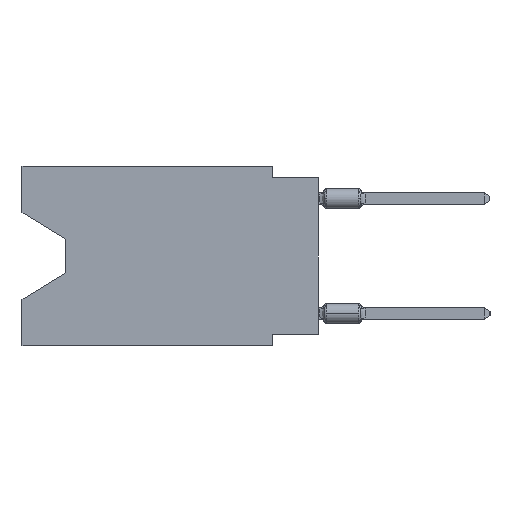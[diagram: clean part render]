
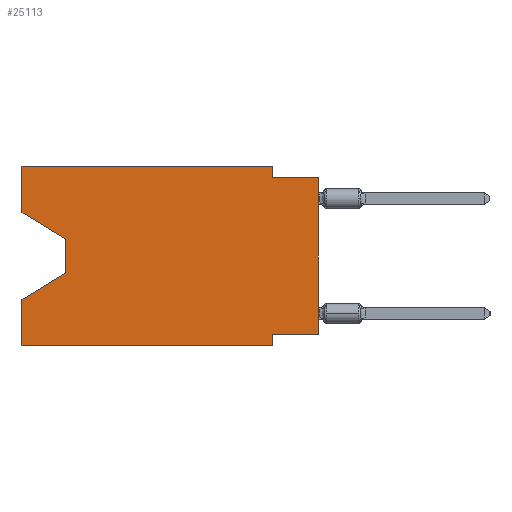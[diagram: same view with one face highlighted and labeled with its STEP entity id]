
A CAD part, left-side view. The second image highlights one B-rep face of the part: STEP entity #25113.
In plain terms, the highlighted planar face has unit normal (-1, 0, 0).
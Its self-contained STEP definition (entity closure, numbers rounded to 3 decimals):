
#298 = LINE ( 'NONE', #15007, #31494 ) ;
#526 = VERTEX_POINT ( 'NONE', #36395 ) ;
#696 = VECTOR ( 'NONE', #44986, 1000. ) ;
#1063 = VECTOR ( 'NONE', #20297, 1000. ) ;
#1226 = DIRECTION ( 'NONE',  ( 0., -1., 0. ) ) ;
#1375 = DIRECTION ( 'NONE',  ( 0., 0., -1. ) ) ;
#2373 = CARTESIAN_POINT ( 'NONE',  ( 0., 16.383, -9.906 ) ) ;
#3007 = LINE ( 'NONE', #8587, #31546 ) ;
#3595 = EDGE_CURVE ( 'NONE', #54115, #43270, #24095, .T. ) ;
#3749 = CARTESIAN_POINT ( 'NONE',  ( 0., 13.97, -4.013 ) ) ;
#4097 = CARTESIAN_POINT ( 'NONE',  ( 0., 16.383, 0. ) ) ;
#4429 = VERTEX_POINT ( 'NONE', #20169 ) ;
#4543 = VERTEX_POINT ( 'NONE', #36067 ) ;
#6307 = EDGE_CURVE ( 'NONE', #28124, #10658, #19996, .T. ) ;
#7804 = EDGE_CURVE ( 'NONE', #526, #4543, #36896, .T. ) ;
#8149 = CARTESIAN_POINT ( 'NONE',  ( 0., 16.383, -7.36 ) ) ;
#8587 = CARTESIAN_POINT ( 'NONE',  ( 0., 13.97, -5.893 ) ) ;
#8866 = VERTEX_POINT ( 'NONE', #20973 ) ;
#9098 = VERTEX_POINT ( 'NONE', #19689 ) ;
#9407 = EDGE_CURVE ( 'NONE', #526, #4429, #37939, .T. ) ;
#10426 = PLANE ( 'NONE',  #21625 ) ;
#10658 = VERTEX_POINT ( 'NONE', #36509 ) ;
#11030 = DIRECTION ( 'NONE',  ( 0., 0., -1. ) ) ;
#11902 = EDGE_CURVE ( 'NONE', #4543, #22830, #56758, .T. ) ;
#13470 = ORIENTED_EDGE ( 'NONE', *, *, #57463, .T. ) ;
#13638 = ORIENTED_EDGE ( 'NONE', *, *, #9407, .T. ) ;
#14748 = VERTEX_POINT ( 'NONE', #20993 ) ;
#15007 = CARTESIAN_POINT ( 'NONE',  ( 0., 2.54, 0. ) ) ;
#16032 = VECTOR ( 'NONE', #37025, 1000. ) ;
#18238 = CARTESIAN_POINT ( 'NONE',  ( 0., 16.383, 0. ) ) ;
#18314 = ORIENTED_EDGE ( 'NONE', *, *, #20501, .F. ) ;
#18347 = CARTESIAN_POINT ( 'NONE',  ( 0., 0., -9.271 ) ) ;
#18638 = CARTESIAN_POINT ( 'NONE',  ( 0., 16.383, -2.546 ) ) ;
#19064 = EDGE_LOOP ( 'NONE', ( #13638, #47439, #13470, #29159, #48305, #47782, #44709, #53096, #45418, #18314, #46433, #48528 ) ) ;
#19689 = CARTESIAN_POINT ( 'NONE',  ( 0., 13.97, -5.893 ) ) ;
#19996 = LINE ( 'NONE', #28891, #1063 ) ;
#20169 = CARTESIAN_POINT ( 'NONE',  ( 0., 13.97, -4.013 ) ) ;
#20297 = DIRECTION ( 'NONE',  ( 0., 0., 1. ) ) ;
#20501 = EDGE_CURVE ( 'NONE', #22830, #8866, #298, .T. ) ;
#20973 = CARTESIAN_POINT ( 'NONE',  ( 0., 2.54, -0.635 ) ) ;
#20993 = CARTESIAN_POINT ( 'NONE',  ( 0., 16.383, -9.906 ) ) ;
#21625 = AXIS2_PLACEMENT_3D ( 'NONE', #43536, #24534, #11030 ) ;
#22146 = CARTESIAN_POINT ( 'NONE',  ( 0., 2.54, -9.271 ) ) ;
#22537 = EDGE_CURVE ( 'NONE', #28124, #54115, #46915, .T. ) ;
#22830 = VERTEX_POINT ( 'NONE', #28356 ) ;
#24095 = LINE ( 'NONE', #29881, #40994 ) ;
#24214 = DIRECTION ( 'NONE',  ( 0., 0., -1. ) ) ;
#24534 = DIRECTION ( 'NONE',  ( 1., 0., 0. ) ) ;
#25113 = ADVANCED_FACE ( 'NONE', ( #33715 ), #10426, .F. ) ;
#26275 = LINE ( 'NONE', #2373, #696 ) ;
#27844 = CARTESIAN_POINT ( 'NONE',  ( 0., 0., -0.635 ) ) ;
#28124 = VERTEX_POINT ( 'NONE', #18347 ) ;
#28356 = CARTESIAN_POINT ( 'NONE',  ( 0., 2.54, 0. ) ) ;
#28633 = VERTEX_POINT ( 'NONE', #8149 ) ;
#28891 = CARTESIAN_POINT ( 'NONE',  ( 0., 0., 0. ) ) ;
#29159 = ORIENTED_EDGE ( 'NONE', *, *, #37665, .F. ) ;
#29357 = VECTOR ( 'NONE', #50683, 1000. ) ;
#29881 = CARTESIAN_POINT ( 'NONE',  ( 0., 2.54, -9.906 ) ) ;
#31494 = VECTOR ( 'NONE', #24214, 1000. ) ;
#31546 = VECTOR ( 'NONE', #55819, 1000. ) ;
#33255 = VECTOR ( 'NONE', #36944, 1000. ) ;
#33715 = FACE_OUTER_BOUND ( 'NONE', #19064, .T. ) ;
#34589 = EDGE_CURVE ( 'NONE', #14748, #43270, #26275, .T. ) ;
#34606 = VECTOR ( 'NONE', #51813, 1000. ) ;
#36067 = CARTESIAN_POINT ( 'NONE',  ( 0., 16.383, 0. ) ) ;
#36395 = CARTESIAN_POINT ( 'NONE',  ( 0., 16.383, -2.546 ) ) ;
#36509 = CARTESIAN_POINT ( 'NONE',  ( 0., 0., -0.635 ) ) ;
#36570 = LINE ( 'NONE', #3749, #29357 ) ;
#36896 = LINE ( 'NONE', #4097, #54079 ) ;
#36944 = DIRECTION ( 'NONE',  ( 0., 0., 1. ) ) ;
#37025 = DIRECTION ( 'NONE',  ( 0., -0.855, -0.519 ) ) ;
#37665 = EDGE_CURVE ( 'NONE', #14748, #28633, #54733, .T. ) ;
#37707 = CARTESIAN_POINT ( 'NONE',  ( 0., 0., -9.271 ) ) ;
#37939 = LINE ( 'NONE', #18638, #16032 ) ;
#37942 = VECTOR ( 'NONE', #51162, 1000. ) ;
#38009 = EDGE_CURVE ( 'NONE', #4429, #9098, #36570, .T. ) ;
#40994 = VECTOR ( 'NONE', #1375, 1000. ) ;
#42833 = EDGE_CURVE ( 'NONE', #8866, #10658, #46548, .T. ) ;
#43270 = VERTEX_POINT ( 'NONE', #56600 ) ;
#43536 = CARTESIAN_POINT ( 'NONE',  ( 0., 16.383, 0. ) ) ;
#44709 = ORIENTED_EDGE ( 'NONE', *, *, #22537, .F. ) ;
#44986 = DIRECTION ( 'NONE',  ( 0., -1., 0. ) ) ;
#45418 = ORIENTED_EDGE ( 'NONE', *, *, #42833, .F. ) ;
#46433 = ORIENTED_EDGE ( 'NONE', *, *, #11902, .F. ) ;
#46548 = LINE ( 'NONE', #27844, #37942 ) ;
#46915 = LINE ( 'NONE', #37707, #34606 ) ;
#47439 = ORIENTED_EDGE ( 'NONE', *, *, #38009, .T. ) ;
#47782 = ORIENTED_EDGE ( 'NONE', *, *, #3595, .F. ) ;
#48305 = ORIENTED_EDGE ( 'NONE', *, *, #34589, .T. ) ;
#48528 = ORIENTED_EDGE ( 'NONE', *, *, #7804, .F. ) ;
#49714 = VECTOR ( 'NONE', #1226, 1000. ) ;
#50683 = DIRECTION ( 'NONE',  ( 0., 0., -1. ) ) ;
#51162 = DIRECTION ( 'NONE',  ( 0., -1., 0. ) ) ;
#51813 = DIRECTION ( 'NONE',  ( 0., 1., 0. ) ) ;
#53042 = CARTESIAN_POINT ( 'NONE',  ( 0., 16.383, 0. ) ) ;
#53096 = ORIENTED_EDGE ( 'NONE', *, *, #6307, .T. ) ;
#54079 = VECTOR ( 'NONE', #59921, 1000. ) ;
#54115 = VERTEX_POINT ( 'NONE', #22146 ) ;
#54733 = LINE ( 'NONE', #18238, #33255 ) ;
#55819 = DIRECTION ( 'NONE',  ( 0., 0.855, -0.519 ) ) ;
#56600 = CARTESIAN_POINT ( 'NONE',  ( 0., 2.54, -9.906 ) ) ;
#56758 = LINE ( 'NONE', #53042, #49714 ) ;
#57463 = EDGE_CURVE ( 'NONE', #9098, #28633, #3007, .T. ) ;
#59921 = DIRECTION ( 'NONE',  ( 0., 0., 1. ) ) ;
